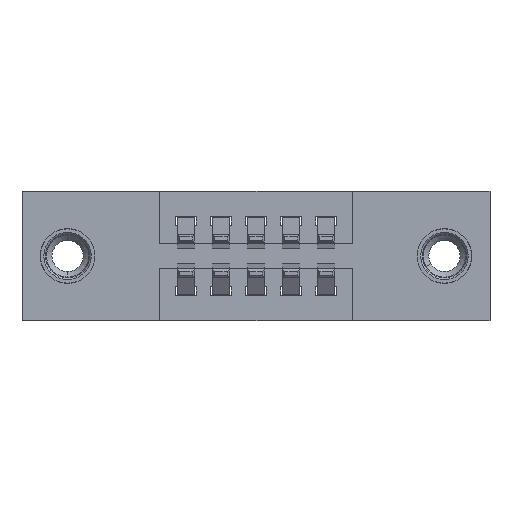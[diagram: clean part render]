
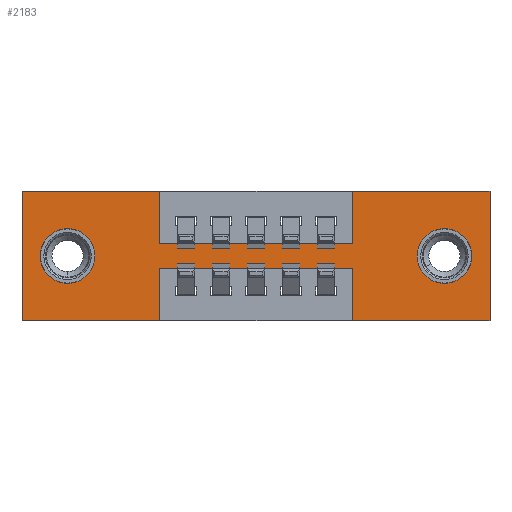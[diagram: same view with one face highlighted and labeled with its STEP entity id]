
A CAD part, front view. The second image highlights one B-rep face of the part: STEP entity #2183.
In plain terms, the highlighted planar face has unit normal (0, -1, 0).
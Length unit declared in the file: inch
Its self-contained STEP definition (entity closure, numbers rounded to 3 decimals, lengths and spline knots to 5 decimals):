
#21 = VERTEX_POINT ( 'NONE', #9974 ) ;
#71 = VERTEX_POINT ( 'NONE', #1374 ) ;
#251 = VERTEX_POINT ( 'NONE', #10062 ) ;
#394 = LINE ( 'NONE', #7169, #4431 ) ;
#400 = DIRECTION ( 'NONE',  ( 0., 0., -1. ) ) ;
#419 = ORIENTED_EDGE ( 'NONE', *, *, #9279, .F. ) ;
#423 = ORIENTED_EDGE ( 'NONE', *, *, #7095, .F. ) ;
#488 = ORIENTED_EDGE ( 'NONE', *, *, #3902, .F. ) ;
#674 = LINE ( 'NONE', #3440, #5210 ) ;
#686 = LINE ( 'NONE', #6825, #9094 ) ;
#690 = DIRECTION ( 'NONE',  ( 0., -1., 0. ) ) ;
#984 = DIRECTION ( 'NONE',  ( 0., 1., 0. ) ) ;
#1140 = LINE ( 'NONE', #6173, #3523 ) ;
#1273 = LINE ( 'NONE', #4057, #3163 ) ;
#1295 = EDGE_CURVE ( 'NONE', #7754, #6804, #4428, .T. ) ;
#1374 = CARTESIAN_POINT ( 'NONE',  ( 0.9425, 0., -0.22 ) ) ;
#1381 = DIRECTION ( 'NONE',  ( 0., 0., 1. ) ) ;
#1437 = LINE ( 'NONE', #8766, #3334 ) ;
#1482 = PLANE ( 'NONE',  #3984 ) ;
#1523 = AXIS2_PLACEMENT_3D ( 'NONE', #5263, #3349, #5251 ) ;
#1556 = CIRCLE ( 'NONE', #1523, 0.078 ) ;
#1567 = VERTEX_POINT ( 'NONE', #3292 ) ;
#1657 = ORIENTED_EDGE ( 'NONE', *, *, #4369, .F. ) ;
#1697 = DIRECTION ( 'NONE',  ( -1., 0., 0. ) ) ;
#1761 = CARTESIAN_POINT ( 'NONE',  ( 0., 0., -0.37 ) ) ;
#1815 = EDGE_CURVE ( 'NONE', #9539, #1567, #1556, .T. ) ;
#1870 = CARTESIAN_POINT ( 'NONE',  ( 0.9425, 0., -0.15 ) ) ;
#2006 = EDGE_LOOP ( 'NONE', ( #6463, #6101, #5684, #6208, #5000, #9760, #1657, #3160, #423, #2480, #488, #419 ) ) ;
#2059 = CARTESIAN_POINT ( 'NONE',  ( 0., 0., 0. ) ) ;
#2116 = CARTESIAN_POINT ( 'NONE',  ( 0.13, 0., -0.185 ) ) ;
#2183 = ADVANCED_FACE ( 'NONE', ( #7092, #2819, #4667 ), #1482, .T. ) ;
#2295 = EDGE_CURVE ( 'NONE', #1567, #9539, #6043, .T. ) ;
#2371 = VERTEX_POINT ( 'NONE', #7248 ) ;
#2409 = VECTOR ( 'NONE', #3810, 39.37008 ) ;
#2427 = VERTEX_POINT ( 'NONE', #1870 ) ;
#2480 = ORIENTED_EDGE ( 'NONE', *, *, #6393, .F. ) ;
#2500 = ORIENTED_EDGE ( 'NONE', *, *, #2295, .T. ) ;
#2583 = VECTOR ( 'NONE', #6942, 39.37008 ) ;
#2598 = CARTESIAN_POINT ( 'NONE',  ( 0.13, 0., -0.263 ) ) ;
#2618 = EDGE_LOOP ( 'NONE', ( #2500, #9151 ) ) ;
#2808 = CARTESIAN_POINT ( 'NONE',  ( 0., 0., 0. ) ) ;
#2809 = CARTESIAN_POINT ( 'NONE',  ( 0.9425, 0., -0.37 ) ) ;
#2819 = FACE_BOUND ( 'NONE', #3096, .T. ) ;
#2820 = DIRECTION ( 'NONE',  ( 1., 0., 0. ) ) ;
#2930 = DIRECTION ( 'NONE',  ( 0., 0., 1. ) ) ;
#3096 = EDGE_LOOP ( 'NONE', ( #4966, #3149 ) ) ;
#3149 = ORIENTED_EDGE ( 'NONE', *, *, #9700, .T. ) ;
#3160 = ORIENTED_EDGE ( 'NONE', *, *, #5456, .F. ) ;
#3161 = CARTESIAN_POINT ( 'NONE',  ( 0.3925, 0., -0.37 ) ) ;
#3163 = VECTOR ( 'NONE', #1697, 39.37008 ) ;
#3192 = CARTESIAN_POINT ( 'NONE',  ( 0.13, 0., -0.107 ) ) ;
#3292 = CARTESIAN_POINT ( 'NONE',  ( 1.205, 0., -0.107 ) ) ;
#3322 = EDGE_CURVE ( 'NONE', #8284, #71, #6683, .T. ) ;
#3334 = VECTOR ( 'NONE', #7294, 39.37008 ) ;
#3349 = DIRECTION ( 'NONE',  ( 0., 1., 0. ) ) ;
#3440 = CARTESIAN_POINT ( 'NONE',  ( 0., 0., -0.37 ) ) ;
#3523 = VECTOR ( 'NONE', #1381, 39.37008 ) ;
#3716 = CARTESIAN_POINT ( 'NONE',  ( 1.205, 0., -0.263 ) ) ;
#3761 = LINE ( 'NONE', #3161, #5651 ) ;
#3810 = DIRECTION ( 'NONE',  ( 0., 0., 1. ) ) ;
#3892 = LINE ( 'NONE', #10144, #9805 ) ;
#3893 = EDGE_CURVE ( 'NONE', #2371, #251, #3761, .T. ) ;
#3902 = EDGE_CURVE ( 'NONE', #9702, #7775, #7573, .T. ) ;
#3972 = CARTESIAN_POINT ( 'NONE',  ( 0., 0., 0. ) ) ;
#3984 = AXIS2_PLACEMENT_3D ( 'NONE', #1761, #690, #9083 ) ;
#4037 = VERTEX_POINT ( 'NONE', #6591 ) ;
#4057 = CARTESIAN_POINT ( 'NONE',  ( 0., 0., -0.37 ) ) ;
#4369 = EDGE_CURVE ( 'NONE', #2427, #7754, #1140, .T. ) ;
#4428 = LINE ( 'NONE', #2808, #2583 ) ;
#4431 = VECTOR ( 'NONE', #6329, 39.37008 ) ;
#4433 = VECTOR ( 'NONE', #400, 39.37008 ) ;
#4667 = FACE_OUTER_BOUND ( 'NONE', #2006, .T. ) ;
#4739 = DIRECTION ( 'NONE',  ( 0., 0., -1. ) ) ;
#4944 = LINE ( 'NONE', #7660, #4433 ) ;
#4966 = ORIENTED_EDGE ( 'NONE', *, *, #5527, .T. ) ;
#5000 = ORIENTED_EDGE ( 'NONE', *, *, #6763, .F. ) ;
#5210 = VECTOR ( 'NONE', #8196, 39.37008 ) ;
#5251 = DIRECTION ( 'NONE',  ( 0., 0., -1. ) ) ;
#5263 = CARTESIAN_POINT ( 'NONE',  ( 1.205, 0., -0.185 ) ) ;
#5406 = VECTOR ( 'NONE', #9391, 39.37008 ) ;
#5456 = EDGE_CURVE ( 'NONE', #6233, #2427, #686, .T. ) ;
#5527 = EDGE_CURVE ( 'NONE', #8630, #8775, #8438, .T. ) ;
#5566 = DIRECTION ( 'NONE',  ( 0., 1., 0. ) ) ;
#5604 = DIRECTION ( 'NONE',  ( 0., 0., -1. ) ) ;
#5651 = VECTOR ( 'NONE', #4739, 39.37008 ) ;
#5684 = ORIENTED_EDGE ( 'NONE', *, *, #3322, .F. ) ;
#5749 = AXIS2_PLACEMENT_3D ( 'NONE', #5774, #984, #6593 ) ;
#5774 = CARTESIAN_POINT ( 'NONE',  ( 0.13, 0., -0.185 ) ) ;
#5909 = EDGE_CURVE ( 'NONE', #4037, #8284, #674, .T. ) ;
#6043 = CIRCLE ( 'NONE', #6711, 0.078 ) ;
#6101 = ORIENTED_EDGE ( 'NONE', *, *, #9235, .F. ) ;
#6173 = CARTESIAN_POINT ( 'NONE',  ( 0.9425, 0., 0. ) ) ;
#6208 = ORIENTED_EDGE ( 'NONE', *, *, #5909, .F. ) ;
#6233 = VERTEX_POINT ( 'NONE', #9206 ) ;
#6329 = DIRECTION ( 'NONE',  ( 1., 0., 0. ) ) ;
#6393 = EDGE_CURVE ( 'NONE', #7775, #21, #394, .T. ) ;
#6463 = ORIENTED_EDGE ( 'NONE', *, *, #3893, .F. ) ;
#6591 = CARTESIAN_POINT ( 'NONE',  ( 1.335, 0., -0.37 ) ) ;
#6593 = DIRECTION ( 'NONE',  ( 0., 0., 1. ) ) ;
#6661 = AXIS2_PLACEMENT_3D ( 'NONE', #2116, #7730, #2930 ) ;
#6683 = LINE ( 'NONE', #2809, #2409 ) ;
#6711 = AXIS2_PLACEMENT_3D ( 'NONE', #6790, #5566, #5604 ) ;
#6757 = CARTESIAN_POINT ( 'NONE',  ( 0.9425, 0., -0.37 ) ) ;
#6763 = EDGE_CURVE ( 'NONE', #6804, #4037, #1437, .T. ) ;
#6790 = CARTESIAN_POINT ( 'NONE',  ( 1.205, 0., -0.185 ) ) ;
#6804 = VERTEX_POINT ( 'NONE', #8793 ) ;
#6825 = CARTESIAN_POINT ( 'NONE',  ( 0.3925, 0., -0.15 ) ) ;
#6942 = DIRECTION ( 'NONE',  ( 1., 0., 0. ) ) ;
#7092 = FACE_BOUND ( 'NONE', #2618, .T. ) ;
#7095 = EDGE_CURVE ( 'NONE', #21, #6233, #4944, .T. ) ;
#7169 = CARTESIAN_POINT ( 'NONE',  ( 0., 0., 0. ) ) ;
#7248 = CARTESIAN_POINT ( 'NONE',  ( 0.3925, 0., -0.22 ) ) ;
#7294 = DIRECTION ( 'NONE',  ( 0., 0., -1. ) ) ;
#7573 = LINE ( 'NONE', #3972, #5406 ) ;
#7650 = CARTESIAN_POINT ( 'NONE',  ( 0.9425, 0., 0. ) ) ;
#7660 = CARTESIAN_POINT ( 'NONE',  ( 0.3925, 0., 0. ) ) ;
#7730 = DIRECTION ( 'NONE',  ( 0., 1., 0. ) ) ;
#7754 = VERTEX_POINT ( 'NONE', #7650 ) ;
#7775 = VERTEX_POINT ( 'NONE', #2059 ) ;
#8196 = DIRECTION ( 'NONE',  ( -1., 0., 0. ) ) ;
#8284 = VERTEX_POINT ( 'NONE', #6757 ) ;
#8438 = CIRCLE ( 'NONE', #6661, 0.078 ) ;
#8630 = VERTEX_POINT ( 'NONE', #3192 ) ;
#8766 = CARTESIAN_POINT ( 'NONE',  ( 1.335, 0., 0. ) ) ;
#8775 = VERTEX_POINT ( 'NONE', #2598 ) ;
#8793 = CARTESIAN_POINT ( 'NONE',  ( 1.335, 0., 0. ) ) ;
#9083 = DIRECTION ( 'NONE',  ( 0., 0., -1. ) ) ;
#9094 = VECTOR ( 'NONE', #2820, 39.37008 ) ;
#9151 = ORIENTED_EDGE ( 'NONE', *, *, #1815, .T. ) ;
#9206 = CARTESIAN_POINT ( 'NONE',  ( 0.3925, 0., -0.15 ) ) ;
#9235 = EDGE_CURVE ( 'NONE', #71, #2371, #3892, .T. ) ;
#9279 = EDGE_CURVE ( 'NONE', #251, #9702, #1273, .T. ) ;
#9335 = CIRCLE ( 'NONE', #5749, 0.078 ) ;
#9391 = DIRECTION ( 'NONE',  ( 0., 0., 1. ) ) ;
#9412 = DIRECTION ( 'NONE',  ( -1., 0., 0. ) ) ;
#9539 = VERTEX_POINT ( 'NONE', #3716 ) ;
#9555 = CARTESIAN_POINT ( 'NONE',  ( 0., 0., -0.37 ) ) ;
#9700 = EDGE_CURVE ( 'NONE', #8775, #8630, #9335, .T. ) ;
#9702 = VERTEX_POINT ( 'NONE', #9555 ) ;
#9760 = ORIENTED_EDGE ( 'NONE', *, *, #1295, .F. ) ;
#9805 = VECTOR ( 'NONE', #9412, 39.37008 ) ;
#9974 = CARTESIAN_POINT ( 'NONE',  ( 0.3925, 0., 0. ) ) ;
#10062 = CARTESIAN_POINT ( 'NONE',  ( 0.3925, 0., -0.37 ) ) ;
#10144 = CARTESIAN_POINT ( 'NONE',  ( 0.3925, 0., -0.22 ) ) ;
